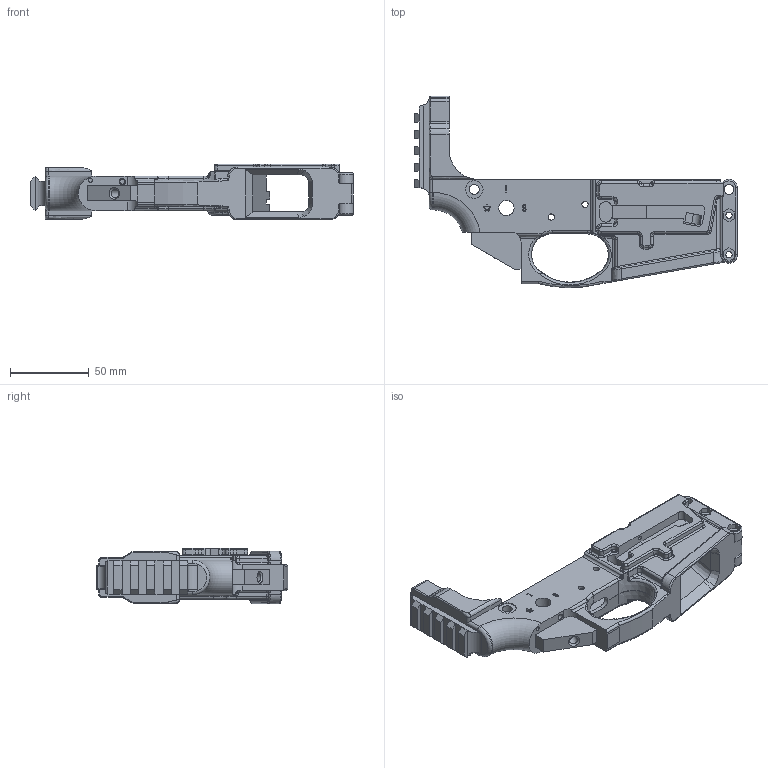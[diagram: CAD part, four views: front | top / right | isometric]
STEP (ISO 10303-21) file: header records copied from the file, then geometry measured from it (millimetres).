
FILE_DESCRIPTION(/* description */ (''),/* implementation_level */ '2;1');
FILE_NAME(/* name */ 'PRM-9.step',/* time_stamp */ '2022-12-27T02:50:47-05:00',/* author */ (''),/* organization */ (''),/* preprocessor_version */ 'ST-DEVELOPER v19.2',/* originating_system */ 'Autodesk Translation Framework v11.17.0.187',/* authorisation */ '');
FILE_SCHEMA (('AUTOMOTIVE_DESIGN { 1 0 10303 214 3 1 1 }'));
Length unit declared in the file: millimetre
Products named in the file (3): Lower Receiver Body; Left Takedown Standoff; Right Takedown Standoff
Assembly tree (2 placements, depth 2):
  Lower Receiver Body
    Left Takedown Standoff
    Right Takedown Standoff
Bounding box: 205.3 x 121.65 x 35.28 mm (x, y, z)
Volume: 163325.8 mm3; surface area: 59786.6 mm2
Topology: 3 solids, 3 shells, 1160 faces, 3148 edges, 2034 vertices
Faces by surface type: plane 637, bspline 269, cylinder 193, torus 46, cone 9, sphere 6
Full cylindrical faces by diameter (mm): 2 x2, 2.464 x1, 2.5 x2, 2.75 x1, 3 x2, 3.2 x1, 3.95 x1, 3.962 x4, 4 x6, 5.35 x1, 6.274 x2, 6.375 x2, 7.3 x2, 9.85 x2, 11.176 x1
Entity records: 42048 total; most frequent: CARTESIAN_POINT 14164, ORIENTED_EDGE 6290, DIRECTION 4911, EDGE_CURVE 3145, LINE 2037, VECTOR 2037, VERTEX_POINT 2034, AXIS2_PLACEMENT_3D 1437
